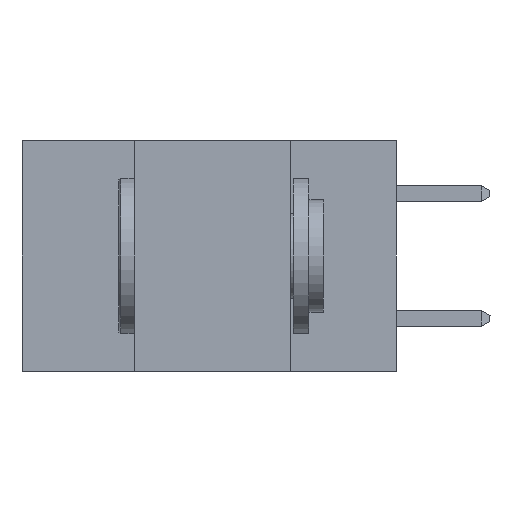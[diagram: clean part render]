
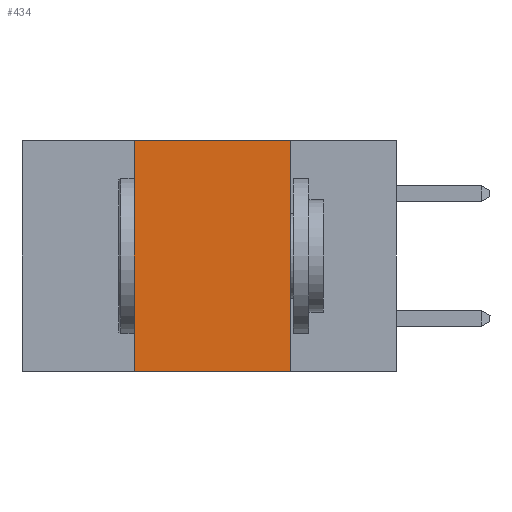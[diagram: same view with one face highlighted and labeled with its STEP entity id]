
A CAD part, left-side view. The second image highlights one B-rep face of the part: STEP entity #434.
In plain terms, the highlighted planar face has unit normal (-1, 0, 0).
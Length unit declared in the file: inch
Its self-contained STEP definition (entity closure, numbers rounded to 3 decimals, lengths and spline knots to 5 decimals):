
#434 = ADVANCED_FACE ( 'NONE', ( #14835 ), #1969, .F. ) ;
#1240 = VERTEX_POINT ( 'NONE', #7313 ) ;
#1969 = PLANE ( 'NONE',  #4836 ) ;
#3138 = VECTOR ( 'NONE', #6777, 39.37008 ) ;
#3447 = VECTOR ( 'NONE', #9993, 39.37008 ) ;
#3535 = CARTESIAN_POINT ( 'NONE',  ( 0., 0.17, -0.37 ) ) ;
#3654 = CARTESIAN_POINT ( 'NONE',  ( 0., 0.42, 0. ) ) ;
#4836 = AXIS2_PLACEMENT_3D ( 'NONE', #14295, #14245, #12328 ) ;
#4955 = VERTEX_POINT ( 'NONE', #3535 ) ;
#5211 = VERTEX_POINT ( 'NONE', #17224 ) ;
#5821 = EDGE_CURVE ( 'NONE', #1240, #4955, #7357, .T. ) ;
#6632 = ORIENTED_EDGE ( 'NONE', *, *, #15602, .T. ) ;
#6759 = CARTESIAN_POINT ( 'NONE',  ( 0., 0.6, 0. ) ) ;
#6777 = DIRECTION ( 'NONE',  ( 0., -1., 0. ) ) ;
#7313 = CARTESIAN_POINT ( 'NONE',  ( 0., 0.17, 0. ) ) ;
#7357 = LINE ( 'NONE', #10056, #3447 ) ;
#7741 = EDGE_CURVE ( 'NONE', #9035, #1240, #17275, .T. ) ;
#8455 = CARTESIAN_POINT ( 'NONE',  ( 0., 0.6, -0.37 ) ) ;
#8752 = CARTESIAN_POINT ( 'NONE',  ( 0., 0.42, -0.37 ) ) ;
#9035 = VERTEX_POINT ( 'NONE', #3654 ) ;
#9681 = EDGE_CURVE ( 'NONE', #5211, #9035, #15235, .T. ) ;
#9993 = DIRECTION ( 'NONE',  ( 0., 0., -1. ) ) ;
#10056 = CARTESIAN_POINT ( 'NONE',  ( 0., 0.17, -0.37 ) ) ;
#11617 = DIRECTION ( 'NONE',  ( 0., 0., 1. ) ) ;
#11862 = ORIENTED_EDGE ( 'NONE', *, *, #7741, .F. ) ;
#12304 = LINE ( 'NONE', #8455, #15762 ) ;
#12327 = ORIENTED_EDGE ( 'NONE', *, *, #5821, .F. ) ;
#12328 = DIRECTION ( 'NONE',  ( 0., 0., -1. ) ) ;
#13895 = EDGE_LOOP ( 'NONE', ( #12327, #11862, #18274, #6632 ) ) ;
#14245 = DIRECTION ( 'NONE',  ( 1., 0., 0. ) ) ;
#14295 = CARTESIAN_POINT ( 'NONE',  ( 0., 0.6, 0. ) ) ;
#14777 = VECTOR ( 'NONE', #11617, 39.37008 ) ;
#14835 = FACE_OUTER_BOUND ( 'NONE', #13895, .T. ) ;
#15235 = LINE ( 'NONE', #8752, #14777 ) ;
#15602 = EDGE_CURVE ( 'NONE', #5211, #4955, #12304, .T. ) ;
#15762 = VECTOR ( 'NONE', #17169, 39.37008 ) ;
#17169 = DIRECTION ( 'NONE',  ( 0., -1., 0. ) ) ;
#17224 = CARTESIAN_POINT ( 'NONE',  ( 0., 0.42, -0.37 ) ) ;
#17275 = LINE ( 'NONE', #6759, #3138 ) ;
#18274 = ORIENTED_EDGE ( 'NONE', *, *, #9681, .F. ) ;
